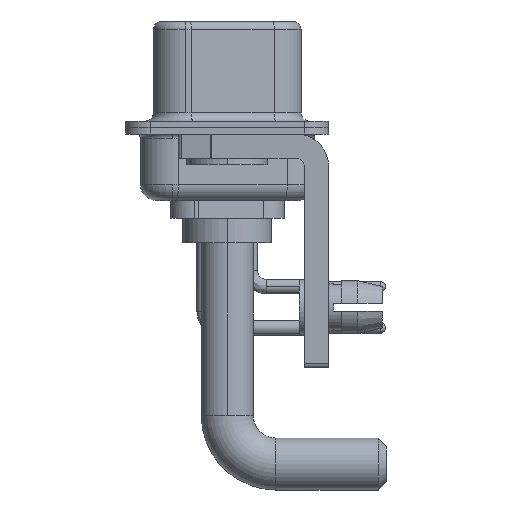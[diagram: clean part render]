
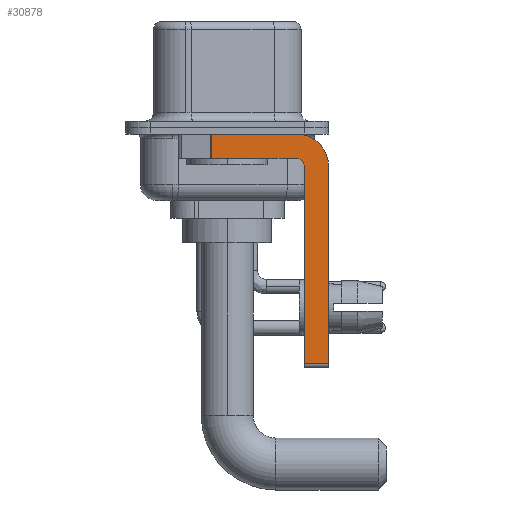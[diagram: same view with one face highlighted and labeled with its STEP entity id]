
A CAD part, left-side view. The second image highlights one B-rep face of the part: STEP entity #30878.
In plain terms, the highlighted planar face has unit normal (-1, 0, 0).
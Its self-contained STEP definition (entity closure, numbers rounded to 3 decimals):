
#210 = CARTESIAN_POINT ( 'NONE',  ( -2.9, -4.25, -1.9 ) ) ;
#445 = VECTOR ( 'NONE', #22715, 1000. ) ;
#767 = AXIS2_PLACEMENT_3D ( 'NONE', #20279, #29829, #8388 ) ;
#1128 = CARTESIAN_POINT ( 'NONE',  ( -2.9, -4.75, -14.8 ) ) ;
#1588 = DIRECTION ( 'NONE',  ( 0., 0., 1. ) ) ;
#1725 = VERTEX_POINT ( 'NONE', #17543 ) ;
#1834 = ORIENTED_EDGE ( 'NONE', *, *, #19978, .T. ) ;
#1857 = CARTESIAN_POINT ( 'NONE',  ( -2.9, -4.75, -14.55 ) ) ;
#1899 = CARTESIAN_POINT ( 'NONE',  ( -2.9, -4.25, -2.4 ) ) ;
#2210 = EDGE_CURVE ( 'NONE', #24412, #15357, #15949, .T. ) ;
#2808 = ORIENTED_EDGE ( 'NONE', *, *, #24851, .F. ) ;
#4094 = CARTESIAN_POINT ( 'NONE',  ( -2.9, 3., -0.4 ) ) ;
#4206 = LINE ( 'NONE', #25800, #14625 ) ;
#5063 = ORIENTED_EDGE ( 'NONE', *, *, #18390, .F. ) ;
#5090 = ORIENTED_EDGE ( 'NONE', *, *, #2210, .T. ) ;
#5228 = VERTEX_POINT ( 'NONE', #210 ) ;
#5331 = CARTESIAN_POINT ( 'NONE',  ( -2.9, -4.25, -1.9 ) ) ;
#5920 = CARTESIAN_POINT ( 'NONE',  ( -2.9, -4.25, -2.4 ) ) ;
#6095 = CARTESIAN_POINT ( 'NONE',  ( -2.9, -4.75, -2.4 ) ) ;
#6229 = CARTESIAN_POINT ( 'NONE',  ( -2.9, -4.25, -0.4 ) ) ;
#6459 = LINE ( 'NONE', #4094, #30414 ) ;
#6878 = LINE ( 'NONE', #1128, #445 ) ;
#7685 = EDGE_CURVE ( 'NONE', #9255, #10577, #23961, .T. ) ;
#8188 = ORIENTED_EDGE ( 'NONE', *, *, #28581, .F. ) ;
#8388 = DIRECTION ( 'NONE',  ( 0., 0., -1. ) ) ;
#9255 = VERTEX_POINT ( 'NONE', #6229 ) ;
#10577 = VERTEX_POINT ( 'NONE', #23257 ) ;
#11594 = DIRECTION ( 'NONE',  ( 0., -1., 0. ) ) ;
#11975 = AXIS2_PLACEMENT_3D ( 'NONE', #5920, #15158, #21870 ) ;
#12229 = LINE ( 'NONE', #5331, #13660 ) ;
#12436 = EDGE_CURVE ( 'NONE', #24412, #9255, #6459, .T. ) ;
#12977 = VERTEX_POINT ( 'NONE', #6095 ) ;
#13479 = DIRECTION ( 'NONE',  ( -1., 0., 0. ) ) ;
#13660 = VECTOR ( 'NONE', #28965, 1000. ) ;
#13769 = VECTOR ( 'NONE', #19497, 1000. ) ;
#14122 = CIRCLE ( 'NONE', #23139, 0.5 ) ;
#14625 = VECTOR ( 'NONE', #19051, 1000. ) ;
#15158 = DIRECTION ( 'NONE',  ( 1., 0., 0. ) ) ;
#15357 = VERTEX_POINT ( 'NONE', #21786 ) ;
#15416 = CARTESIAN_POINT ( 'NONE',  ( -2.9, 0.978, -0.4 ) ) ;
#15765 = FACE_OUTER_BOUND ( 'NONE', #27737, .T. ) ;
#15949 = LINE ( 'NONE', #25493, #26688 ) ;
#17543 = CARTESIAN_POINT ( 'NONE',  ( -2.9, -6.25, -14.55 ) ) ;
#17699 = ORIENTED_EDGE ( 'NONE', *, *, #30725, .F. ) ;
#18330 = ORIENTED_EDGE ( 'NONE', *, *, #12436, .F. ) ;
#18390 = EDGE_CURVE ( 'NONE', #12977, #5228, #14122, .T. ) ;
#19051 = DIRECTION ( 'NONE',  ( 0., -1., 0. ) ) ;
#19497 = DIRECTION ( 'NONE',  ( 0., 0., -1. ) ) ;
#19978 = EDGE_CURVE ( 'NONE', #30496, #1725, #4206, .T. ) ;
#20279 = CARTESIAN_POINT ( 'NONE',  ( -2.9, -4.25, -2.4 ) ) ;
#21684 = CARTESIAN_POINT ( 'NONE',  ( -2.9, -6.25, -2.4 ) ) ;
#21786 = CARTESIAN_POINT ( 'NONE',  ( -2.9, 0.978, -1.9 ) ) ;
#21870 = DIRECTION ( 'NONE',  ( 0., 0., -1. ) ) ;
#22715 = DIRECTION ( 'NONE',  ( 0., 0., 1. ) ) ;
#23139 = AXIS2_PLACEMENT_3D ( 'NONE', #1899, #13479, #1588 ) ;
#23257 = CARTESIAN_POINT ( 'NONE',  ( -2.9, -6.25, -2.4 ) ) ;
#23961 = CIRCLE ( 'NONE', #11975, 2. ) ;
#24412 = VERTEX_POINT ( 'NONE', #15416 ) ;
#24851 = EDGE_CURVE ( 'NONE', #30496, #12977, #6878, .T. ) ;
#25183 = DIRECTION ( 'NONE',  ( 0., 0., -1. ) ) ;
#25300 = PLANE ( 'NONE',  #767 ) ;
#25493 = CARTESIAN_POINT ( 'NONE',  ( -2.9, 0.978, -1.9 ) ) ;
#25800 = CARTESIAN_POINT ( 'NONE',  ( -2.9, -4.25, -14.55 ) ) ;
#26247 = LINE ( 'NONE', #21684, #13769 ) ;
#26688 = VECTOR ( 'NONE', #25183, 1000. ) ;
#27737 = EDGE_LOOP ( 'NONE', ( #18330, #5090, #8188, #5063, #2808, #1834, #17699, #29109 ) ) ;
#28581 = EDGE_CURVE ( 'NONE', #5228, #15357, #12229, .T. ) ;
#28965 = DIRECTION ( 'NONE',  ( 0., 1., 0. ) ) ;
#29109 = ORIENTED_EDGE ( 'NONE', *, *, #7685, .F. ) ;
#29829 = DIRECTION ( 'NONE',  ( 1., 0., 0. ) ) ;
#30414 = VECTOR ( 'NONE', #11594, 1000. ) ;
#30496 = VERTEX_POINT ( 'NONE', #1857 ) ;
#30725 = EDGE_CURVE ( 'NONE', #10577, #1725, #26247, .T. ) ;
#30878 = ADVANCED_FACE ( 'NONE', ( #15765 ), #25300, .F. ) ;
